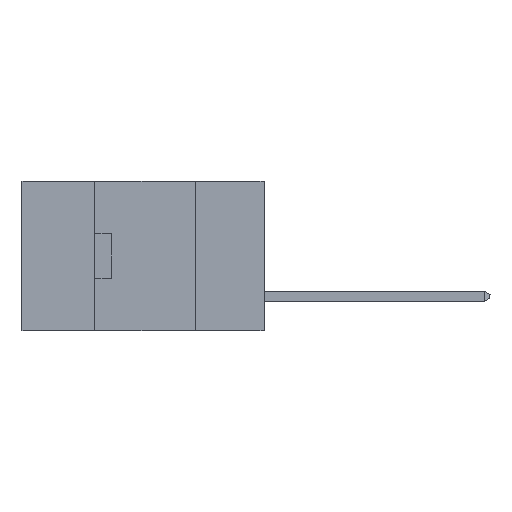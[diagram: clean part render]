
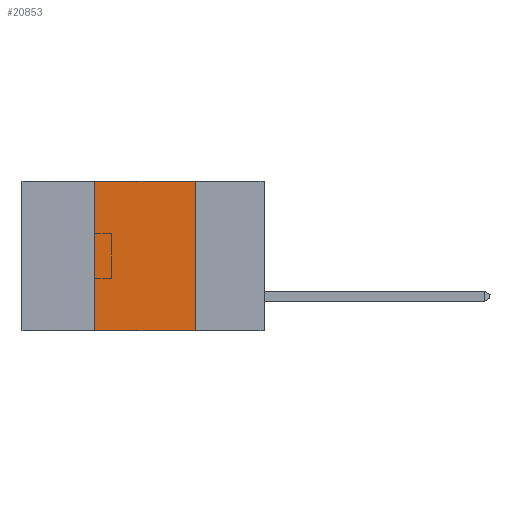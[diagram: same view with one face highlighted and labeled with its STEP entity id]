
A CAD part, left-side view. The second image highlights one B-rep face of the part: STEP entity #20853.
In plain terms, the highlighted planar face has unit normal (-1, 0, 0).
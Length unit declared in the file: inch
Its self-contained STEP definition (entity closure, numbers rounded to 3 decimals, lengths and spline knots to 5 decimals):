
#210 = CARTESIAN_POINT ( 'NONE',  ( 0., 0.17, -0.37 ) ) ;
#303 = CARTESIAN_POINT ( 'NONE',  ( 0., 0.17, -0.37 ) ) ;
#372 = ORIENTED_EDGE ( 'NONE', *, *, #23716, .F. ) ;
#880 = VECTOR ( 'NONE', #13046, 39.37008 ) ;
#1057 = FACE_OUTER_BOUND ( 'NONE', #11681, .T. ) ;
#2328 = AXIS2_PLACEMENT_3D ( 'NONE', #15955, #26236, #7639 ) ;
#2741 = CARTESIAN_POINT ( 'NONE',  ( 0., 0.17, 0. ) ) ;
#4345 = VECTOR ( 'NONE', #9008, 39.37008 ) ;
#4889 = LINE ( 'NONE', #13220, #4345 ) ;
#5650 = VECTOR ( 'NONE', #15056, 39.37008 ) ;
#6010 = CARTESIAN_POINT ( 'NONE',  ( 0., 0.42, -0.37 ) ) ;
#6709 = LINE ( 'NONE', #303, #5650 ) ;
#7639 = DIRECTION ( 'NONE',  ( 0., 0., -1. ) ) ;
#7860 = ORIENTED_EDGE ( 'NONE', *, *, #23176, .F. ) ;
#8981 = LINE ( 'NONE', #17300, #880 ) ;
#9008 = DIRECTION ( 'NONE',  ( 0., 0., 1. ) ) ;
#9388 = CARTESIAN_POINT ( 'NONE',  ( 0., 0.6, 0. ) ) ;
#9401 = PLANE ( 'NONE',  #2328 ) ;
#10578 = VECTOR ( 'NONE', #11285, 39.37008 ) ;
#11037 = CARTESIAN_POINT ( 'NONE',  ( 0., 0.42, 0. ) ) ;
#11285 = DIRECTION ( 'NONE',  ( 0., -1., 0. ) ) ;
#11529 = VERTEX_POINT ( 'NONE', #2741 ) ;
#11681 = EDGE_LOOP ( 'NONE', ( #7860, #16122, #372, #23396 ) ) ;
#13046 = DIRECTION ( 'NONE',  ( 0., -1., 0. ) ) ;
#13220 = CARTESIAN_POINT ( 'NONE',  ( 0., 0.42, -0.37 ) ) ;
#15056 = DIRECTION ( 'NONE',  ( 0., 0., -1. ) ) ;
#15955 = CARTESIAN_POINT ( 'NONE',  ( 0., 0.6, 0. ) ) ;
#16122 = ORIENTED_EDGE ( 'NONE', *, *, #19768, .F. ) ;
#16917 = VERTEX_POINT ( 'NONE', #210 ) ;
#17300 = CARTESIAN_POINT ( 'NONE',  ( 0., 0.6, -0.37 ) ) ;
#19768 = EDGE_CURVE ( 'NONE', #22386, #11529, #24416, .T. ) ;
#20853 = ADVANCED_FACE ( 'NONE', ( #1057 ), #9401, .F. ) ;
#22185 = VERTEX_POINT ( 'NONE', #6010 ) ;
#22386 = VERTEX_POINT ( 'NONE', #11037 ) ;
#23176 = EDGE_CURVE ( 'NONE', #11529, #16917, #6709, .T. ) ;
#23396 = ORIENTED_EDGE ( 'NONE', *, *, #24152, .T. ) ;
#23716 = EDGE_CURVE ( 'NONE', #22185, #22386, #4889, .T. ) ;
#24152 = EDGE_CURVE ( 'NONE', #22185, #16917, #8981, .T. ) ;
#24416 = LINE ( 'NONE', #9388, #10578 ) ;
#26236 = DIRECTION ( 'NONE',  ( 1., 0., 0. ) ) ;
